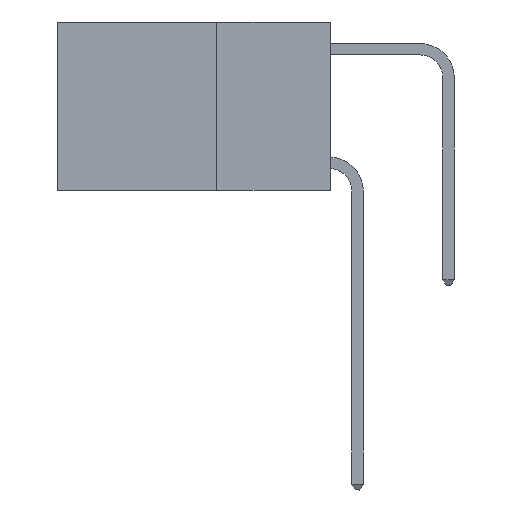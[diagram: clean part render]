
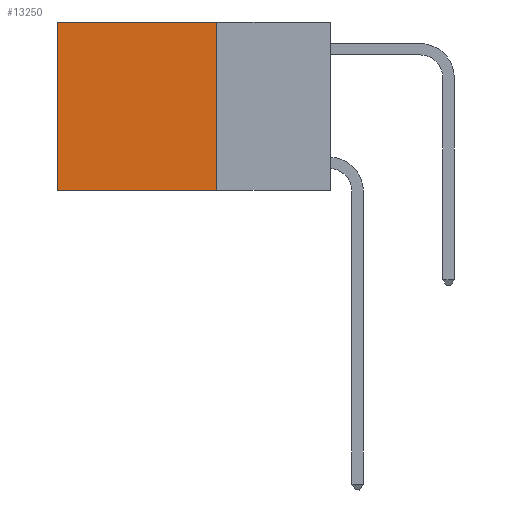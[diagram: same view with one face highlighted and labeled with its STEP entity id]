
A CAD part, left-side view. The second image highlights one B-rep face of the part: STEP entity #13250.
In plain terms, the highlighted planar face has unit normal (-1, 0, 0).
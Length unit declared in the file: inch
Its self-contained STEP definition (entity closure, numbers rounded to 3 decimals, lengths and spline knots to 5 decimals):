
#369 = CARTESIAN_POINT ( 'NONE',  ( 0.2625, 0.6, 0. ) ) ;
#1201 = EDGE_LOOP ( 'NONE', ( #15612, #6810, #16349, #5340 ) ) ;
#1227 = CARTESIAN_POINT ( 'NONE',  ( 0.2625, 0.25, 0. ) ) ;
#1623 = LINE ( 'NONE', #4353, #9352 ) ;
#1695 = DIRECTION ( 'NONE',  ( 0., 1., 0. ) ) ;
#1850 = LINE ( 'NONE', #18667, #9578 ) ;
#2422 = VECTOR ( 'NONE', #5668, 39.37008 ) ;
#2790 = AXIS2_PLACEMENT_3D ( 'NONE', #1227, #9000, #19842 ) ;
#3539 = VERTEX_POINT ( 'NONE', #3828 ) ;
#3828 = CARTESIAN_POINT ( 'NONE',  ( 0.2625, 0.6, 0. ) ) ;
#4117 = CARTESIAN_POINT ( 'NONE',  ( 0.2625, 0.25, 0. ) ) ;
#4353 = CARTESIAN_POINT ( 'NONE',  ( 0.2625, 0.25, 0. ) ) ;
#5340 = ORIENTED_EDGE ( 'NONE', *, *, #10981, .T. ) ;
#5668 = DIRECTION ( 'NONE',  ( 0., 1., 0. ) ) ;
#6810 = ORIENTED_EDGE ( 'NONE', *, *, #14034, .F. ) ;
#7193 = FACE_OUTER_BOUND ( 'NONE', #1201, .T. ) ;
#8659 = EDGE_CURVE ( 'NONE', #3539, #11226, #15331, .T. ) ;
#8917 = DIRECTION ( 'NONE',  ( 0., 0., -1. ) ) ;
#9000 = DIRECTION ( 'NONE',  ( 1., 0., 0. ) ) ;
#9352 = VECTOR ( 'NONE', #8917, 39.37008 ) ;
#9578 = VECTOR ( 'NONE', #1695, 39.37008 ) ;
#10245 = CARTESIAN_POINT ( 'NONE',  ( 0.2625, 0.25, -0.37 ) ) ;
#10981 = EDGE_CURVE ( 'NONE', #17918, #3539, #14730, .T. ) ;
#11226 = VERTEX_POINT ( 'NONE', #12362 ) ;
#11227 = DIRECTION ( 'NONE',  ( 0., 0., -1. ) ) ;
#12362 = CARTESIAN_POINT ( 'NONE',  ( 0.2625, 0.6, -0.37 ) ) ;
#13247 = CARTESIAN_POINT ( 'NONE',  ( 0.2625, 0.25, 0. ) ) ;
#13250 = ADVANCED_FACE ( 'NONE', ( #7193 ), #18278, .F. ) ;
#13816 = EDGE_CURVE ( 'NONE', #17918, #14377, #1623, .T. ) ;
#14034 = EDGE_CURVE ( 'NONE', #14377, #11226, #1850, .T. ) ;
#14377 = VERTEX_POINT ( 'NONE', #10245 ) ;
#14730 = LINE ( 'NONE', #4117, #2422 ) ;
#15331 = LINE ( 'NONE', #369, #18954 ) ;
#15612 = ORIENTED_EDGE ( 'NONE', *, *, #8659, .T. ) ;
#16349 = ORIENTED_EDGE ( 'NONE', *, *, #13816, .F. ) ;
#17918 = VERTEX_POINT ( 'NONE', #13247 ) ;
#18278 = PLANE ( 'NONE',  #2790 ) ;
#18667 = CARTESIAN_POINT ( 'NONE',  ( 0.2625, 0.25, -0.37 ) ) ;
#18954 = VECTOR ( 'NONE', #11227, 39.37008 ) ;
#19842 = DIRECTION ( 'NONE',  ( 0., 0., -1. ) ) ;
